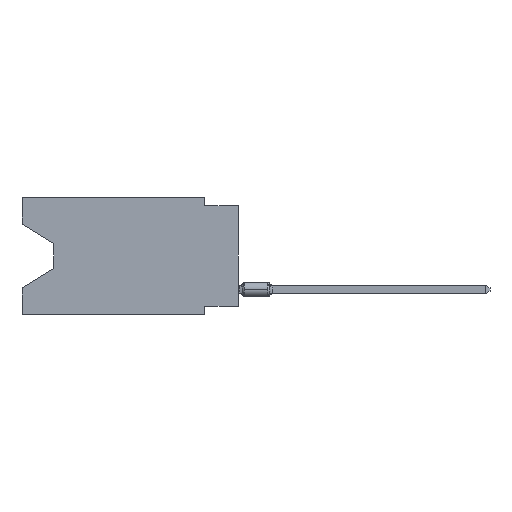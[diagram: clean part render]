
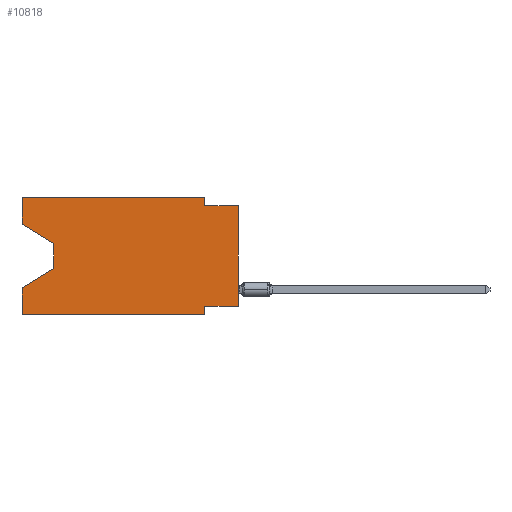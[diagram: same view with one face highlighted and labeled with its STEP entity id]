
A CAD part, left-side view. The second image highlights one B-rep face of the part: STEP entity #10818.
In plain terms, the highlighted planar face has unit normal (-1, 0, 0).
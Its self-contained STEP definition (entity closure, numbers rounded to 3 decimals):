
#348 = CARTESIAN_POINT ( 'NONE',  ( 0., 16.383, -8.89 ) ) ;
#439 = VECTOR ( 'NONE', #1534, 1000. ) ;
#497 = EDGE_CURVE ( 'NONE', #2439, #14482, #11500, .T. ) ;
#832 = VERTEX_POINT ( 'NONE', #11358 ) ;
#1228 = CARTESIAN_POINT ( 'NONE',  ( 0., 2.54, 0. ) ) ;
#1500 = CARTESIAN_POINT ( 'NONE',  ( 0., 13.97, -5.385 ) ) ;
#1534 = DIRECTION ( 'NONE',  ( 0., 0., 1. ) ) ;
#1550 = CARTESIAN_POINT ( 'NONE',  ( 0., 16.383, 0. ) ) ;
#1551 = DIRECTION ( 'NONE',  ( 0., 0., -1. ) ) ;
#1857 = LINE ( 'NONE', #6246, #10826 ) ;
#1970 = ORIENTED_EDGE ( 'NONE', *, *, #14768, .F. ) ;
#2439 = VERTEX_POINT ( 'NONE', #16594 ) ;
#2718 = VERTEX_POINT ( 'NONE', #348 ) ;
#2800 = DIRECTION ( 'NONE',  ( 0., 0., -1. ) ) ;
#2851 = LINE ( 'NONE', #14712, #5154 ) ;
#2903 = VECTOR ( 'NONE', #1551, 1000. ) ;
#3045 = EDGE_CURVE ( 'NONE', #14482, #21452, #15630, .T. ) ;
#3138 = CARTESIAN_POINT ( 'NONE',  ( 0., 16.383, 0. ) ) ;
#3226 = VECTOR ( 'NONE', #17749, 1000. ) ;
#4301 = VECTOR ( 'NONE', #16136, 1000. ) ;
#4391 = CARTESIAN_POINT ( 'NONE',  ( 0., 2.54, -8.255 ) ) ;
#4446 = CARTESIAN_POINT ( 'NONE',  ( 0., 16.383, -6.852 ) ) ;
#4741 = EDGE_CURVE ( 'NONE', #832, #17527, #1857, .T. ) ;
#5107 = LINE ( 'NONE', #8794, #439 ) ;
#5154 = VECTOR ( 'NONE', #9648, 1000. ) ;
#5532 = VERTEX_POINT ( 'NONE', #4446 ) ;
#5711 = LINE ( 'NONE', #12518, #9150 ) ;
#6246 = CARTESIAN_POINT ( 'NONE',  ( 0., 13.97, -3.505 ) ) ;
#6261 = VECTOR ( 'NONE', #12412, 1000. ) ;
#6307 = CARTESIAN_POINT ( 'NONE',  ( 0., 16.383, 0. ) ) ;
#6539 = EDGE_CURVE ( 'NONE', #10422, #21827, #19305, .T. ) ;
#6589 = PLANE ( 'NONE',  #17430 ) ;
#6922 = EDGE_CURVE ( 'NONE', #18688, #11359, #2851, .T. ) ;
#6990 = DIRECTION ( 'NONE',  ( 0., -0.855, -0.519 ) ) ;
#7052 = LINE ( 'NONE', #9335, #4301 ) ;
#7904 = CARTESIAN_POINT ( 'NONE',  ( 0., 2.54, -0.635 ) ) ;
#8094 = EDGE_CURVE ( 'NONE', #18688, #21827, #5107, .T. ) ;
#8238 = CARTESIAN_POINT ( 'NONE',  ( 0., 2.54, -8.89 ) ) ;
#8280 = DIRECTION ( 'NONE',  ( 0., 0., 1. ) ) ;
#8414 = EDGE_CURVE ( 'NONE', #17527, #5532, #22458, .T. ) ;
#8794 = CARTESIAN_POINT ( 'NONE',  ( 0., 0., 0. ) ) ;
#8899 = CARTESIAN_POINT ( 'NONE',  ( 0., 16.383, 0. ) ) ;
#9150 = VECTOR ( 'NONE', #6990, 1000. ) ;
#9223 = ORIENTED_EDGE ( 'NONE', *, *, #16050, .F. ) ;
#9335 = CARTESIAN_POINT ( 'NONE',  ( 0., 2.54, 0. ) ) ;
#9648 = DIRECTION ( 'NONE',  ( 0., 1., 0. ) ) ;
#9987 = CARTESIAN_POINT ( 'NONE',  ( 0., 16.383, -8.89 ) ) ;
#10134 = CARTESIAN_POINT ( 'NONE',  ( 0., 2.54, -8.89 ) ) ;
#10327 = VECTOR ( 'NONE', #15155, 1000. ) ;
#10422 = VERTEX_POINT ( 'NONE', #7904 ) ;
#10739 = LINE ( 'NONE', #8899, #3226 ) ;
#10818 = ADVANCED_FACE ( 'NONE', ( #19454 ), #6589, .F. ) ;
#10822 = DIRECTION ( 'NONE',  ( 1., 0., 0. ) ) ;
#10826 = VECTOR ( 'NONE', #2800, 1000. ) ;
#11031 = ORIENTED_EDGE ( 'NONE', *, *, #3045, .F. ) ;
#11358 = CARTESIAN_POINT ( 'NONE',  ( 0., 13.97, -3.505 ) ) ;
#11359 = VERTEX_POINT ( 'NONE', #4391 ) ;
#11500 = LINE ( 'NONE', #6307, #13100 ) ;
#12412 = DIRECTION ( 'NONE',  ( 0., -1., 0. ) ) ;
#12518 = CARTESIAN_POINT ( 'NONE',  ( 0., 16.383, -2.038 ) ) ;
#12618 = EDGE_LOOP ( 'NONE', ( #18268, #21010, #13955, #9223, #17868, #14394, #21151, #15117, #13420, #1970, #11031, #19009 ) ) ;
#13100 = VECTOR ( 'NONE', #8280, 1000. ) ;
#13420 = ORIENTED_EDGE ( 'NONE', *, *, #6539, .F. ) ;
#13632 = CARTESIAN_POINT ( 'NONE',  ( 0., 0., -8.255 ) ) ;
#13955 = ORIENTED_EDGE ( 'NONE', *, *, #8414, .T. ) ;
#14394 = ORIENTED_EDGE ( 'NONE', *, *, #17087, .F. ) ;
#14482 = VERTEX_POINT ( 'NONE', #1550 ) ;
#14576 = CARTESIAN_POINT ( 'NONE',  ( 0., 0., -0.635 ) ) ;
#14712 = CARTESIAN_POINT ( 'NONE',  ( 0., 0., -8.255 ) ) ;
#14768 = EDGE_CURVE ( 'NONE', #21452, #10422, #7052, .T. ) ;
#15117 = ORIENTED_EDGE ( 'NONE', *, *, #8094, .T. ) ;
#15155 = DIRECTION ( 'NONE',  ( 0., -1., 0. ) ) ;
#15630 = LINE ( 'NONE', #20808, #20834 ) ;
#16050 = EDGE_CURVE ( 'NONE', #2718, #5532, #10739, .T. ) ;
#16136 = DIRECTION ( 'NONE',  ( 0., 0., -1. ) ) ;
#16290 = VERTEX_POINT ( 'NONE', #10134 ) ;
#16594 = CARTESIAN_POINT ( 'NONE',  ( 0., 16.383, -2.038 ) ) ;
#16767 = EDGE_CURVE ( 'NONE', #2439, #832, #5711, .T. ) ;
#17087 = EDGE_CURVE ( 'NONE', #11359, #16290, #17321, .T. ) ;
#17227 = LINE ( 'NONE', #9987, #10327 ) ;
#17321 = LINE ( 'NONE', #8238, #2903 ) ;
#17430 = AXIS2_PLACEMENT_3D ( 'NONE', #3138, #10822, #17833 ) ;
#17527 = VERTEX_POINT ( 'NONE', #21059 ) ;
#17749 = DIRECTION ( 'NONE',  ( 0., 0., 1. ) ) ;
#17833 = DIRECTION ( 'NONE',  ( 0., 0., -1. ) ) ;
#17868 = ORIENTED_EDGE ( 'NONE', *, *, #20118, .T. ) ;
#18268 = ORIENTED_EDGE ( 'NONE', *, *, #16767, .T. ) ;
#18688 = VERTEX_POINT ( 'NONE', #13632 ) ;
#19009 = ORIENTED_EDGE ( 'NONE', *, *, #497, .F. ) ;
#19305 = LINE ( 'NONE', #14576, #6261 ) ;
#19454 = FACE_OUTER_BOUND ( 'NONE', #12618, .T. ) ;
#20118 = EDGE_CURVE ( 'NONE', #2718, #16290, #17227, .T. ) ;
#20613 = DIRECTION ( 'NONE',  ( 0., 0.855, -0.519 ) ) ;
#20808 = CARTESIAN_POINT ( 'NONE',  ( 0., 16.383, 0. ) ) ;
#20834 = VECTOR ( 'NONE', #22658, 1000. ) ;
#21010 = ORIENTED_EDGE ( 'NONE', *, *, #4741, .T. ) ;
#21059 = CARTESIAN_POINT ( 'NONE',  ( 0., 13.97, -5.385 ) ) ;
#21151 = ORIENTED_EDGE ( 'NONE', *, *, #6922, .F. ) ;
#21452 = VERTEX_POINT ( 'NONE', #1228 ) ;
#21738 = VECTOR ( 'NONE', #20613, 1000. ) ;
#21827 = VERTEX_POINT ( 'NONE', #22619 ) ;
#22458 = LINE ( 'NONE', #1500, #21738 ) ;
#22619 = CARTESIAN_POINT ( 'NONE',  ( 0., 0., -0.635 ) ) ;
#22658 = DIRECTION ( 'NONE',  ( 0., -1., 0. ) ) ;
